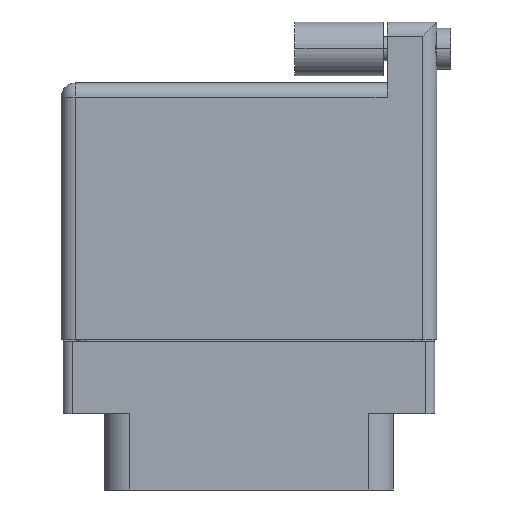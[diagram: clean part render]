
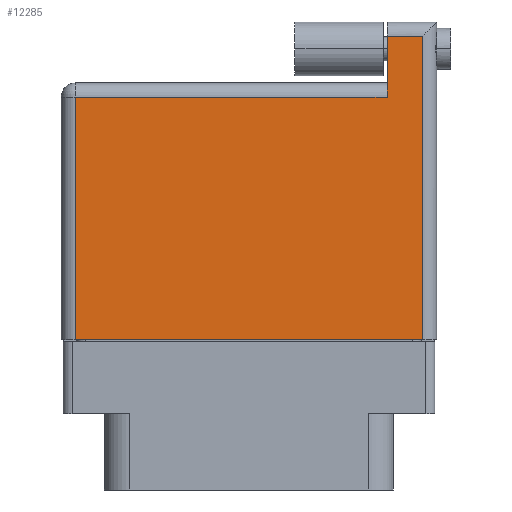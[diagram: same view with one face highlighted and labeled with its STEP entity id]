
A CAD part, front view. The second image highlights one B-rep face of the part: STEP entity #12285.
In plain terms, the highlighted face is planar.
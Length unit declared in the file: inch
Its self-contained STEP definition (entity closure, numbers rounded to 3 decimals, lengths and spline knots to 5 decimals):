
#291 = VERTEX_POINT ( 'NONE', #9617 ) ;
#886 = VERTEX_POINT ( 'NONE', #3288 ) ;
#3229 = VECTOR ( 'NONE', #21563, 39.37008 ) ;
#3288 = CARTESIAN_POINT ( 'NONE',  ( 0.4875, 0.97, 0.3575 ) ) ;
#3547 = CARTESIAN_POINT ( 'NONE',  ( 0.6125, 0.97, 0.3575 ) ) ;
#3720 = VECTOR ( 'NONE', #15836, 39.37008 ) ;
#4492 = VERTEX_POINT ( 'NONE', #3547 ) ;
#5180 = CARTESIAN_POINT ( 'NONE',  ( -0.6125, -0.1, 0.3575 ) ) ;
#5690 = LINE ( 'NONE', #16358, #15845 ) ;
#6533 = CARTESIAN_POINT ( 'NONE',  ( -0.6125, 0.756, 0.3575 ) ) ;
#8173 = EDGE_CURVE ( 'NONE', #4492, #886, #24766, .T. ) ;
#8187 = VERTEX_POINT ( 'NONE', #5180 ) ;
#8246 = EDGE_CURVE ( 'NONE', #291, #10518, #25394, .T. ) ;
#9021 = VECTOR ( 'NONE', #19709, 39.37008 ) ;
#9050 = FACE_OUTER_BOUND ( 'NONE', #15169, .T. ) ;
#9409 = EDGE_CURVE ( 'NONE', #886, #291, #24425, .T. ) ;
#9617 = CARTESIAN_POINT ( 'NONE',  ( 0.4875, 0.756, 0.3575 ) ) ;
#9644 = DIRECTION ( 'NONE',  ( 0., -1., 0. ) ) ;
#9878 = CARTESIAN_POINT ( 'NONE',  ( 0.6125, 1.02, 0.3575 ) ) ;
#10305 = ORIENTED_EDGE ( 'NONE', *, *, #9409, .T. ) ;
#10518 = VERTEX_POINT ( 'NONE', #6533 ) ;
#12099 = VECTOR ( 'NONE', #9644, 39.37008 ) ;
#12285 = ADVANCED_FACE ( 'NONE', ( #9050 ), #23554, .F. ) ;
#12558 = ORIENTED_EDGE ( 'NONE', *, *, #13364, .T. ) ;
#12834 = CARTESIAN_POINT ( 'NONE',  ( 0.6125, -0.1, 0.3575 ) ) ;
#13103 = CARTESIAN_POINT ( 'NONE',  ( -0.6625, -0.1, 0.3575 ) ) ;
#13364 = EDGE_CURVE ( 'NONE', #10518, #8187, #5690, .T. ) ;
#13669 = CARTESIAN_POINT ( 'NONE',  ( -0.6625, 0.756, 0.3575 ) ) ;
#14410 = LINE ( 'NONE', #9878, #9021 ) ;
#15169 = EDGE_LOOP ( 'NONE', ( #15480, #24522, #16392, #10305, #15812, #12558 ) ) ;
#15480 = ORIENTED_EDGE ( 'NONE', *, *, #22798, .T. ) ;
#15812 = ORIENTED_EDGE ( 'NONE', *, *, #8246, .T. ) ;
#15836 = DIRECTION ( 'NONE',  ( 1., 0., 0. ) ) ;
#15845 = VECTOR ( 'NONE', #22344, 39.37008 ) ;
#16358 = CARTESIAN_POINT ( 'NONE',  ( -0.6125, -0.1, 0.3575 ) ) ;
#16392 = ORIENTED_EDGE ( 'NONE', *, *, #8173, .T. ) ;
#17247 = EDGE_CURVE ( 'NONE', #17714, #4492, #14410, .T. ) ;
#17714 = VERTEX_POINT ( 'NONE', #12834 ) ;
#17740 = CARTESIAN_POINT ( 'NONE',  ( -0.6625, 0.806, 0.3575 ) ) ;
#18042 = DIRECTION ( 'NONE',  ( -1., 0., 0. ) ) ;
#18487 = AXIS2_PLACEMENT_3D ( 'NONE', #17740, #21883, #21542 ) ;
#18657 = LINE ( 'NONE', #13103, #3720 ) ;
#19709 = DIRECTION ( 'NONE',  ( 0., 1., 0. ) ) ;
#20057 = VECTOR ( 'NONE', #18042, 39.37008 ) ;
#21542 = DIRECTION ( 'NONE',  ( -1., 0., 0. ) ) ;
#21563 = DIRECTION ( 'NONE',  ( -1., 0., 0. ) ) ;
#21769 = CARTESIAN_POINT ( 'NONE',  ( 0.4875, 1.02, 0.3575 ) ) ;
#21883 = DIRECTION ( 'NONE',  ( 0., 0., -1. ) ) ;
#22344 = DIRECTION ( 'NONE',  ( 0., -1., 0. ) ) ;
#22798 = EDGE_CURVE ( 'NONE', #8187, #17714, #18657, .T. ) ;
#23554 = PLANE ( 'NONE',  #18487 ) ;
#24425 = LINE ( 'NONE', #21769, #12099 ) ;
#24522 = ORIENTED_EDGE ( 'NONE', *, *, #17247, .T. ) ;
#24766 = LINE ( 'NONE', #25604, #3229 ) ;
#25394 = LINE ( 'NONE', #13669, #20057 ) ;
#25604 = CARTESIAN_POINT ( 'NONE',  ( -0.6625, 0.97, 0.3575 ) ) ;
